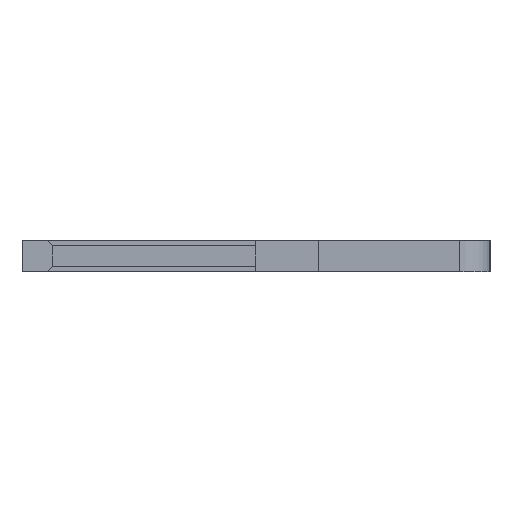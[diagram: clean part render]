
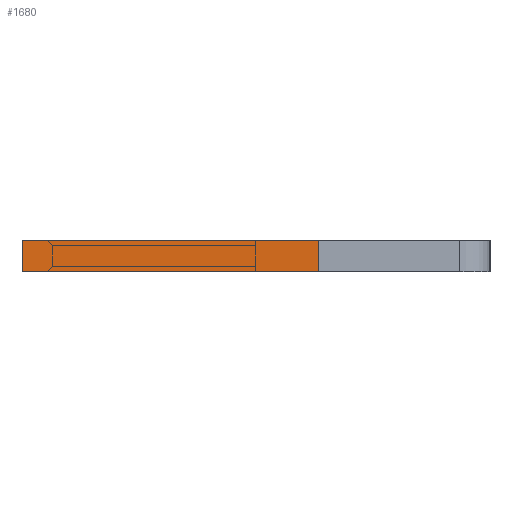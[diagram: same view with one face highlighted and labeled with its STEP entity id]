
A CAD part, left-side view. The second image highlights one B-rep face of the part: STEP entity #1680.
In plain terms, the highlighted face is planar.
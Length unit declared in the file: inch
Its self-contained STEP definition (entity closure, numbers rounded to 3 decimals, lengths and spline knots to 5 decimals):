
#35 = ORIENTED_EDGE ( 'NONE', *, *, #1192, .F. ) ;
#91 = VERTEX_POINT ( 'NONE', #1784 ) ;
#142 = DIRECTION ( 'NONE',  ( 0., 1., 0. ) ) ;
#246 = LINE ( 'NONE', #1602, #2021 ) ;
#356 = CARTESIAN_POINT ( 'NONE',  ( 0.01, 0.15, -0.04 ) ) ;
#435 = VECTOR ( 'NONE', #1870, 39.37008 ) ;
#631 = AXIS2_PLACEMENT_3D ( 'NONE', #356, #2214, #1993 ) ;
#819 = DIRECTION ( 'NONE',  ( -1., 0., 0. ) ) ;
#832 = EDGE_CURVE ( 'NONE', #1942, #1361, #2059, .T. ) ;
#943 = VECTOR ( 'NONE', #142, 39.37008 ) ;
#945 = CARTESIAN_POINT ( 'NONE',  ( 0.01, 0.15, -0.04 ) ) ;
#970 = PLANE ( 'NONE',  #631 ) ;
#1010 = CARTESIAN_POINT ( 'NONE',  ( 0.01, 0.15, -0.04 ) ) ;
#1024 = CARTESIAN_POINT ( 'NONE',  ( 0.01, -0.04, -0.04 ) ) ;
#1065 = LINE ( 'NONE', #945, #943 ) ;
#1079 = CARTESIAN_POINT ( 'NONE',  ( -0.01, -0.04, -0.04 ) ) ;
#1192 = EDGE_CURVE ( 'NONE', #91, #2201, #2480, .T. ) ;
#1269 = ORIENTED_EDGE ( 'NONE', *, *, #1929, .F. ) ;
#1361 = VERTEX_POINT ( 'NONE', #1079 ) ;
#1430 = DIRECTION ( 'NONE',  ( 0., 1., 0. ) ) ;
#1462 = ORIENTED_EDGE ( 'NONE', *, *, #2292, .T. ) ;
#1465 = EDGE_LOOP ( 'NONE', ( #1462, #35, #1269, #2301 ) ) ;
#1602 = CARTESIAN_POINT ( 'NONE',  ( -0.01, 0.15, -0.04 ) ) ;
#1608 = CARTESIAN_POINT ( 'NONE',  ( -0.01, 0.15, -0.04 ) ) ;
#1612 = VECTOR ( 'NONE', #819, 39.37008 ) ;
#1680 = ADVANCED_FACE ( 'NONE', ( #1774 ), #970, .F. ) ;
#1774 = FACE_OUTER_BOUND ( 'NONE', #1465, .T. ) ;
#1784 = CARTESIAN_POINT ( 'NONE',  ( 0.01, 0.15, -0.04 ) ) ;
#1790 = CARTESIAN_POINT ( 'NONE',  ( 0.01, -0.04, -0.04 ) ) ;
#1870 = DIRECTION ( 'NONE',  ( -1., 0., 0. ) ) ;
#1929 = EDGE_CURVE ( 'NONE', #1942, #91, #1065, .T. ) ;
#1942 = VERTEX_POINT ( 'NONE', #1790 ) ;
#1993 = DIRECTION ( 'NONE',  ( 1., 0., 0. ) ) ;
#2021 = VECTOR ( 'NONE', #1430, 39.37008 ) ;
#2059 = LINE ( 'NONE', #1024, #435 ) ;
#2201 = VERTEX_POINT ( 'NONE', #1608 ) ;
#2214 = DIRECTION ( 'NONE',  ( 0., 0., 1. ) ) ;
#2292 = EDGE_CURVE ( 'NONE', #1361, #2201, #246, .T. ) ;
#2301 = ORIENTED_EDGE ( 'NONE', *, *, #832, .T. ) ;
#2480 = LINE ( 'NONE', #1010, #1612 ) ;
